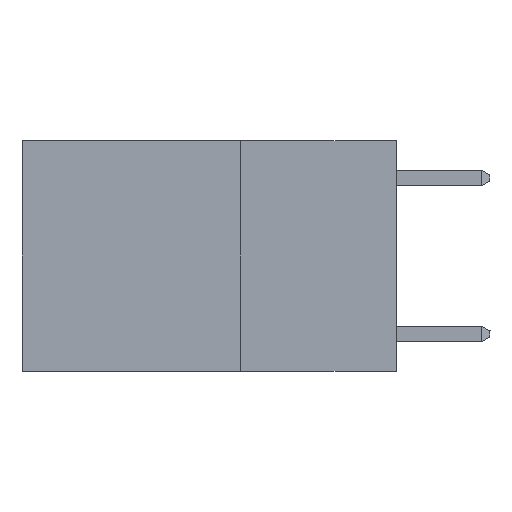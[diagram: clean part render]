
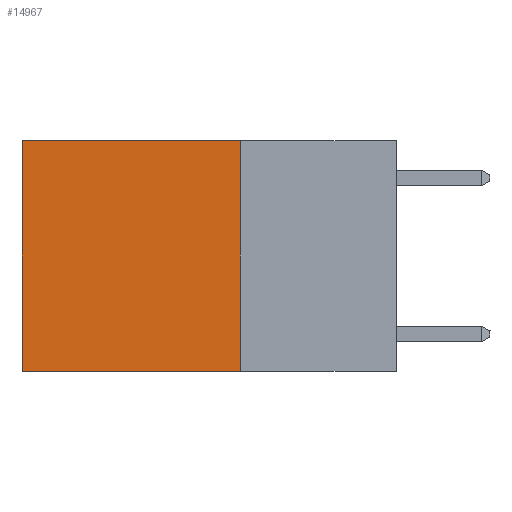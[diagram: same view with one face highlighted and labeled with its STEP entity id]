
A CAD part, left-side view. The second image highlights one B-rep face of the part: STEP entity #14967.
In plain terms, the highlighted planar face has unit normal (-1, 0, 0).
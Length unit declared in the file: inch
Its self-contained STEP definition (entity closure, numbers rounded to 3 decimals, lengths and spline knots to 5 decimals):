
#796 = FACE_OUTER_BOUND ( 'NONE', #16652, .T. ) ;
#1275 = CARTESIAN_POINT ( 'NONE',  ( 0.2625, 0.25, 0. ) ) ;
#1383 = DIRECTION ( 'NONE',  ( 0., 0., -1. ) ) ;
#1514 = VERTEX_POINT ( 'NONE', #12564 ) ;
#1770 = CARTESIAN_POINT ( 'NONE',  ( 0.2625, 0.25, 0. ) ) ;
#3995 = VECTOR ( 'NONE', #22724, 39.37008 ) ;
#4822 = ORIENTED_EDGE ( 'NONE', *, *, #14992, .T. ) ;
#6151 = LINE ( 'NONE', #23978, #17461 ) ;
#6466 = ORIENTED_EDGE ( 'NONE', *, *, #25123, .F. ) ;
#7534 = VERTEX_POINT ( 'NONE', #1770 ) ;
#8563 = CARTESIAN_POINT ( 'NONE',  ( 0.2625, 0.6, -0.37 ) ) ;
#8973 = AXIS2_PLACEMENT_3D ( 'NONE', #1275, #14951, #1383 ) ;
#9674 = EDGE_CURVE ( 'NONE', #7534, #20095, #20277, .T. ) ;
#11111 = VERTEX_POINT ( 'NONE', #8563 ) ;
#12458 = CARTESIAN_POINT ( 'NONE',  ( 0.2625, 0.25, 0. ) ) ;
#12564 = CARTESIAN_POINT ( 'NONE',  ( 0.2625, 0.6, 0. ) ) ;
#13600 = VECTOR ( 'NONE', #28450, 39.37008 ) ;
#13693 = CARTESIAN_POINT ( 'NONE',  ( 0.2625, 0.25, -0.37 ) ) ;
#14951 = DIRECTION ( 'NONE',  ( 1., 0., 0. ) ) ;
#14967 = ADVANCED_FACE ( 'NONE', ( #796 ), #21619, .F. ) ;
#14992 = EDGE_CURVE ( 'NONE', #1514, #11111, #6151, .T. ) ;
#15048 = DIRECTION ( 'NONE',  ( 0., 0., -1. ) ) ;
#15648 = ORIENTED_EDGE ( 'NONE', *, *, #9674, .F. ) ;
#16652 = EDGE_LOOP ( 'NONE', ( #4822, #6466, #15648, #26865 ) ) ;
#17431 = LINE ( 'NONE', #13693, #3995 ) ;
#17461 = VECTOR ( 'NONE', #15048, 39.37008 ) ;
#19704 = CARTESIAN_POINT ( 'NONE',  ( 0.2625, 0.25, 0. ) ) ;
#20095 = VERTEX_POINT ( 'NONE', #23200 ) ;
#20277 = LINE ( 'NONE', #19704, #13600 ) ;
#21619 = PLANE ( 'NONE',  #8973 ) ;
#21912 = EDGE_CURVE ( 'NONE', #7534, #1514, #25932, .T. ) ;
#22724 = DIRECTION ( 'NONE',  ( 0., 1., 0. ) ) ;
#23200 = CARTESIAN_POINT ( 'NONE',  ( 0.2625, 0.25, -0.37 ) ) ;
#23650 = DIRECTION ( 'NONE',  ( 0., 1., 0. ) ) ;
#23978 = CARTESIAN_POINT ( 'NONE',  ( 0.2625, 0.6, 0. ) ) ;
#25123 = EDGE_CURVE ( 'NONE', #20095, #11111, #17431, .T. ) ;
#25258 = VECTOR ( 'NONE', #23650, 39.37008 ) ;
#25932 = LINE ( 'NONE', #12458, #25258 ) ;
#26865 = ORIENTED_EDGE ( 'NONE', *, *, #21912, .T. ) ;
#28450 = DIRECTION ( 'NONE',  ( 0., 0., -1. ) ) ;
